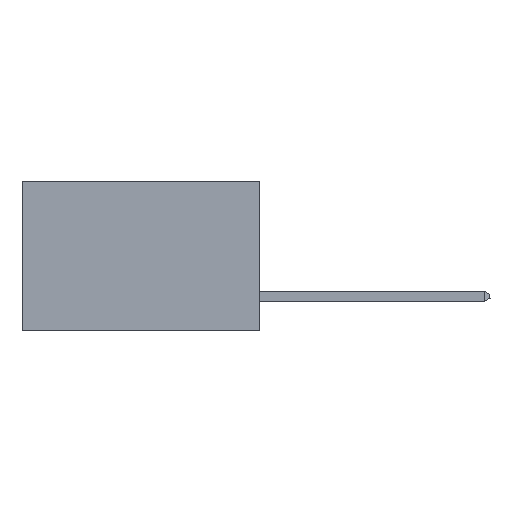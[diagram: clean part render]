
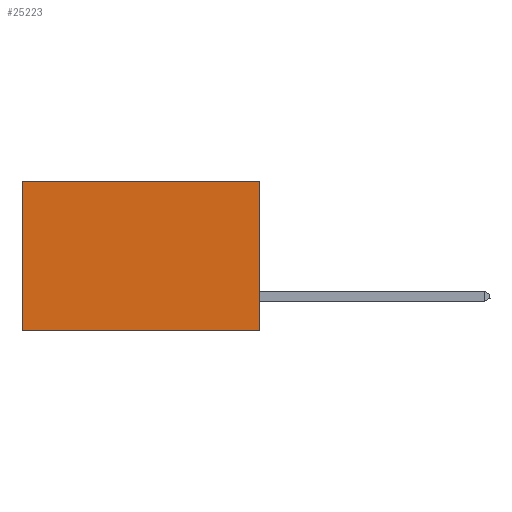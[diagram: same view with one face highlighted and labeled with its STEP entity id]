
A CAD part, left-side view. The second image highlights one B-rep face of the part: STEP entity #25223.
In plain terms, the highlighted planar face has unit normal (-1, 0, 0).
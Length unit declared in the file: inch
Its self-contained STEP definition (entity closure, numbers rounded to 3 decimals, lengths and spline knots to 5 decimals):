
#527 = DIRECTION ( 'NONE',  ( 0., 0., -1. ) ) ;
#684 = ORIENTED_EDGE ( 'NONE', *, *, #10206, .T. ) ;
#687 = CARTESIAN_POINT ( 'NONE',  ( 0.277, 0.59, -0.37 ) ) ;
#1333 = VECTOR ( 'NONE', #2029, 39.37008 ) ;
#1664 = CARTESIAN_POINT ( 'NONE',  ( 0.277, 0., 0. ) ) ;
#2029 = DIRECTION ( 'NONE',  ( 0., 1., 0. ) ) ;
#7401 = ORIENTED_EDGE ( 'NONE', *, *, #21184, .F. ) ;
#7453 = LINE ( 'NONE', #1664, #17595 ) ;
#9399 = DIRECTION ( 'NONE',  ( 0., 0., -1. ) ) ;
#9762 = FACE_OUTER_BOUND ( 'NONE', #18924, .T. ) ;
#10196 = VERTEX_POINT ( 'NONE', #20065 ) ;
#10206 = EDGE_CURVE ( 'NONE', #11532, #19286, #25724, .T. ) ;
#11532 = VERTEX_POINT ( 'NONE', #18279 ) ;
#12508 = CARTESIAN_POINT ( 'NONE',  ( 0.277, 0., -0.37 ) ) ;
#13437 = DIRECTION ( 'NONE',  ( 1., 0., 0. ) ) ;
#13916 = AXIS2_PLACEMENT_3D ( 'NONE', #21965, #13437, #527 ) ;
#14419 = VECTOR ( 'NONE', #9399, 39.37008 ) ;
#14715 = DIRECTION ( 'NONE',  ( 0., 0., -1. ) ) ;
#15574 = PLANE ( 'NONE',  #13916 ) ;
#15825 = EDGE_CURVE ( 'NONE', #23539, #11532, #7453, .T. ) ;
#16378 = VECTOR ( 'NONE', #14715, 39.37008 ) ;
#16449 = EDGE_CURVE ( 'NONE', #10196, #19286, #18561, .T. ) ;
#17595 = VECTOR ( 'NONE', #18912, 39.37008 ) ;
#18263 = CARTESIAN_POINT ( 'NONE',  ( 0.277, 0., 0. ) ) ;
#18279 = CARTESIAN_POINT ( 'NONE',  ( 0.277, 0.59, 0. ) ) ;
#18326 = CARTESIAN_POINT ( 'NONE',  ( 0.277, 0.59, -0.37 ) ) ;
#18561 = LINE ( 'NONE', #27614, #1333 ) ;
#18631 = ORIENTED_EDGE ( 'NONE', *, *, #16449, .F. ) ;
#18912 = DIRECTION ( 'NONE',  ( 0., 1., 0. ) ) ;
#18924 = EDGE_LOOP ( 'NONE', ( #684, #18631, #7401, #19503 ) ) ;
#19286 = VERTEX_POINT ( 'NONE', #18326 ) ;
#19503 = ORIENTED_EDGE ( 'NONE', *, *, #15825, .T. ) ;
#20065 = CARTESIAN_POINT ( 'NONE',  ( 0.277, 0., -0.37 ) ) ;
#21184 = EDGE_CURVE ( 'NONE', #23539, #10196, #22666, .T. ) ;
#21965 = CARTESIAN_POINT ( 'NONE',  ( 0.277, 0., -0.37 ) ) ;
#22666 = LINE ( 'NONE', #12508, #16378 ) ;
#23539 = VERTEX_POINT ( 'NONE', #18263 ) ;
#25223 = ADVANCED_FACE ( 'NONE', ( #9762 ), #15574, .F. ) ;
#25724 = LINE ( 'NONE', #687, #14419 ) ;
#27614 = CARTESIAN_POINT ( 'NONE',  ( 0.277, 0., -0.37 ) ) ;
